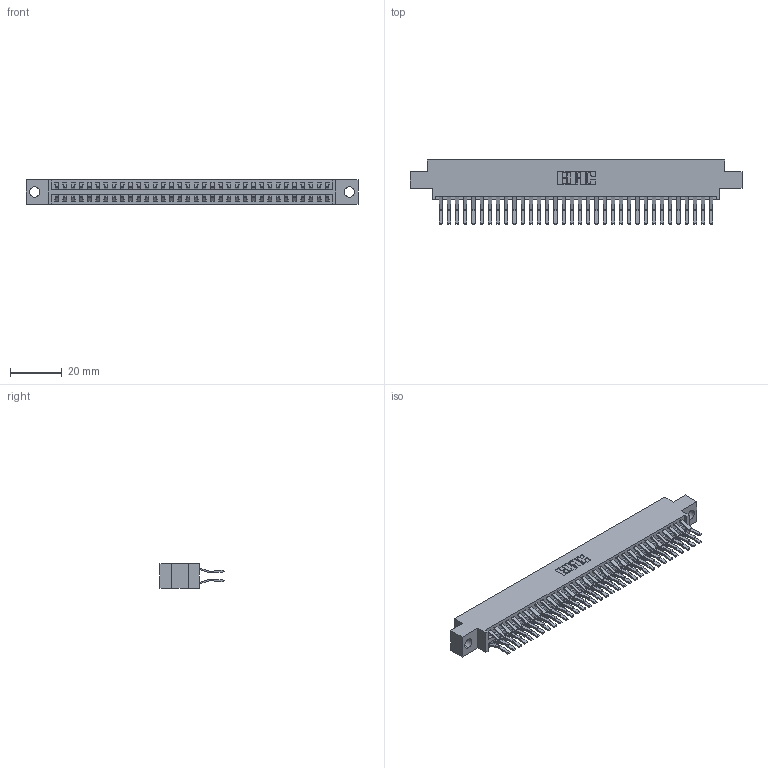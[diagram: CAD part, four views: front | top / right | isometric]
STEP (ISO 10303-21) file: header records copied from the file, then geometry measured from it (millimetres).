
FILE_DESCRIPTION (( 'STEP AP203' ), '1' );
FILE_NAME ('346-068-560-804.STEP', '2018-08-28T22:40:07', ( '' ), ( '' ), 'SwSTEP 2.0', 'SolidWorks 2016', '' );
FILE_SCHEMA (( 'CONFIG_CONTROL_DESIGN' ));
Length unit declared in the file: inch
Products named in the file (3): 346-068-560-804; 346 Part_0.170 Offset - 0.156 Dia-TH; 345-292-001_560 Tail
Assembly tree (69 placements, depth 2):
  346-068-560-804
    346 Part_0.170 Offset - 0.156 Dia-TH
    345-292-001_560 Tail  x68
Bounding box: 128.52 x 24.78 x 9.4 mm (x, y, z)
Volume: 12673.8 mm3; surface area: 18477.4 mm2
Topology: 69 solids, 69 shells, 3798 faces, 11289 edges, 7434 vertices
Faces by surface type: plane 2460, cylinder 1338
Entity records: 23489 total; most frequent: CARTESIAN_POINT 3884, ORIENTED_EDGE 3818, DIRECTION 3477, EDGE_CURVE 1909, LINE 1637, VECTOR 1637, VERTEX_POINT 1270, AXIS2_PLACEMENT_3D 920
